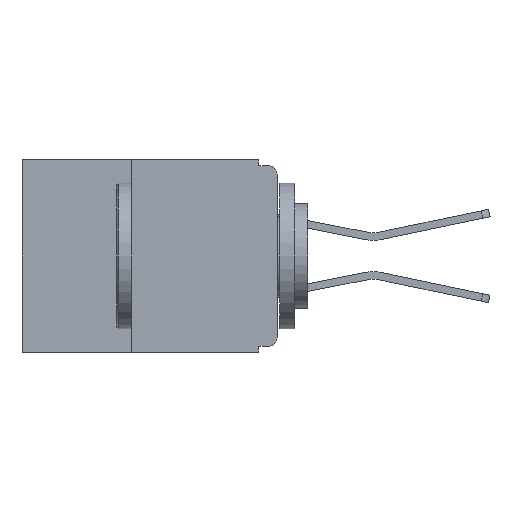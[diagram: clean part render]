
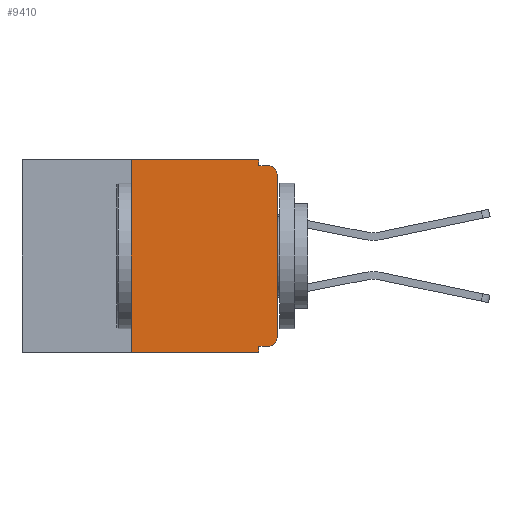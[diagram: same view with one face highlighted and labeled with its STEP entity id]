
A CAD part, left-side view. The second image highlights one B-rep face of the part: STEP entity #9410.
In plain terms, the highlighted planar face has unit normal (-1, 0, 0).
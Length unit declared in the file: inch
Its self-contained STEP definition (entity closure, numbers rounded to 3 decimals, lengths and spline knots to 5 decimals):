
#22 = VECTOR ( 'NONE', #3259, 39.37008 ) ;
#170 = VERTEX_POINT ( 'NONE', #4362 ) ;
#253 = DIRECTION ( 'NONE',  ( 0., 0., -1. ) ) ;
#289 = DIRECTION ( 'NONE',  ( 0., 1., 0. ) ) ;
#506 = VERTEX_POINT ( 'NONE', #2105 ) ;
#507 = EDGE_CURVE ( 'NONE', #8969, #3438, #7579, .T. ) ;
#522 = DIRECTION ( 'NONE',  ( 1., 0., 0. ) ) ;
#640 = EDGE_CURVE ( 'NONE', #170, #8969, #14253, .T. ) ;
#646 = ORIENTED_EDGE ( 'NONE', *, *, #10496, .F. ) ;
#837 = ORIENTED_EDGE ( 'NONE', *, *, #13535, .T. ) ;
#1074 = CARTESIAN_POINT ( 'NONE',  ( 0., 0.031, 0. ) ) ;
#1313 = VERTEX_POINT ( 'NONE', #2822 ) ;
#1616 = ORIENTED_EDGE ( 'NONE', *, *, #4049, .T. ) ;
#1804 = CARTESIAN_POINT ( 'NONE',  ( 0., 0.25, 0. ) ) ;
#1896 = DIRECTION ( 'NONE',  ( 0., 0., 1. ) ) ;
#2105 = CARTESIAN_POINT ( 'NONE',  ( 0., 0.031, -0.32 ) ) ;
#2135 = EDGE_CURVE ( 'NONE', #5074, #9166, #2692, .T. ) ;
#2250 = ORIENTED_EDGE ( 'NONE', *, *, #2135, .T. ) ;
#2692 = CIRCLE ( 'NONE', #13013, 0.015 ) ;
#2728 = PLANE ( 'NONE',  #12878 ) ;
#2822 = CARTESIAN_POINT ( 'NONE',  ( 0., 0.015, -0.01 ) ) ;
#2914 = LINE ( 'NONE', #4872, #8069 ) ;
#2948 = ORIENTED_EDGE ( 'NONE', *, *, #507, .F. ) ;
#3066 = LINE ( 'NONE', #5465, #22 ) ;
#3076 = CARTESIAN_POINT ( 'NONE',  ( 0., 0.031, -0.01 ) ) ;
#3259 = DIRECTION ( 'NONE',  ( 0., 0., -1. ) ) ;
#3438 = VERTEX_POINT ( 'NONE', #1074 ) ;
#3751 = DIRECTION ( 'NONE',  ( 0., -1., 0. ) ) ;
#3814 = CARTESIAN_POINT ( 'NONE',  ( 0., 0.015, -0.305 ) ) ;
#4049 = EDGE_CURVE ( 'NONE', #9166, #13528, #13084, .T. ) ;
#4107 = LINE ( 'NONE', #7011, #6673 ) ;
#4362 = CARTESIAN_POINT ( 'NONE',  ( 0., 0.25, -0.33 ) ) ;
#4366 = ORIENTED_EDGE ( 'NONE', *, *, #640, .F. ) ;
#4523 = ORIENTED_EDGE ( 'NONE', *, *, #6803, .F. ) ;
#4835 = VERTEX_POINT ( 'NONE', #3076 ) ;
#4872 = CARTESIAN_POINT ( 'NONE',  ( 0., 0.437, -0.33 ) ) ;
#5035 = CARTESIAN_POINT ( 'NONE',  ( 0., 0.437, 0. ) ) ;
#5074 = VERTEX_POINT ( 'NONE', #5640 ) ;
#5465 = CARTESIAN_POINT ( 'NONE',  ( 0., 0.031, 0. ) ) ;
#5545 = VECTOR ( 'NONE', #1896, 39.37008 ) ;
#5640 = CARTESIAN_POINT ( 'NONE',  ( 0., 0.015, -0.32 ) ) ;
#5930 = EDGE_CURVE ( 'NONE', #3438, #4835, #3066, .T. ) ;
#6469 = VECTOR ( 'NONE', #9945, 39.37008 ) ;
#6673 = VECTOR ( 'NONE', #289, 39.37008 ) ;
#6803 = EDGE_CURVE ( 'NONE', #5074, #506, #4107, .T. ) ;
#6806 = LINE ( 'NONE', #9896, #6469 ) ;
#6982 = DIRECTION ( 'NONE',  ( -1., 0., 0. ) ) ;
#7011 = CARTESIAN_POINT ( 'NONE',  ( 0., 0., -0.32 ) ) ;
#7251 = VECTOR ( 'NONE', #8173, 39.37008 ) ;
#7579 = LINE ( 'NONE', #10080, #13081 ) ;
#7591 = ORIENTED_EDGE ( 'NONE', *, *, #5930, .F. ) ;
#7895 = CARTESIAN_POINT ( 'NONE',  ( 0., 0., -0.01 ) ) ;
#8069 = VECTOR ( 'NONE', #3751, 39.37008 ) ;
#8170 = VECTOR ( 'NONE', #9019, 39.37008 ) ;
#8173 = DIRECTION ( 'NONE',  ( 0., 0., 1. ) ) ;
#8320 = DIRECTION ( 'NONE',  ( 0., 0., -1. ) ) ;
#8385 = EDGE_CURVE ( 'NONE', #506, #12043, #6806, .T. ) ;
#8523 = LINE ( 'NONE', #7895, #8170 ) ;
#8678 = EDGE_LOOP ( 'NONE', ( #1616, #11404, #646, #7591, #2948, #4366, #837, #13991, #4523, #2250 ) ) ;
#8726 = CARTESIAN_POINT ( 'NONE',  ( 0., 0.031, -0.33 ) ) ;
#8924 = DIRECTION ( 'NONE',  ( 0., -1., 0. ) ) ;
#8969 = VERTEX_POINT ( 'NONE', #1804 ) ;
#9019 = DIRECTION ( 'NONE',  ( 0., -1., 0. ) ) ;
#9166 = VERTEX_POINT ( 'NONE', #13366 ) ;
#9326 = DIRECTION ( 'NONE',  ( -1., 0., 0. ) ) ;
#9410 = ADVANCED_FACE ( 'NONE', ( #10919 ), #2728, .F. ) ;
#9510 = CARTESIAN_POINT ( 'NONE',  ( 0., 0.25, -0.33 ) ) ;
#9665 = DIRECTION ( 'NONE',  ( 0., 0., -1. ) ) ;
#9896 = CARTESIAN_POINT ( 'NONE',  ( 0., 0.031, -0.33 ) ) ;
#9945 = DIRECTION ( 'NONE',  ( 0., 0., -1. ) ) ;
#10080 = CARTESIAN_POINT ( 'NONE',  ( 0., 0.437, 0. ) ) ;
#10496 = EDGE_CURVE ( 'NONE', #4835, #1313, #8523, .T. ) ;
#10919 = FACE_OUTER_BOUND ( 'NONE', #8678, .T. ) ;
#11404 = ORIENTED_EDGE ( 'NONE', *, *, #11756, .T. ) ;
#11434 = CARTESIAN_POINT ( 'NONE',  ( 0., 0., -0.025 ) ) ;
#11756 = EDGE_CURVE ( 'NONE', #13528, #1313, #14302, .T. ) ;
#12043 = VERTEX_POINT ( 'NONE', #8726 ) ;
#12878 = AXIS2_PLACEMENT_3D ( 'NONE', #5035, #522, #8320 ) ;
#13013 = AXIS2_PLACEMENT_3D ( 'NONE', #3814, #9326, #9665 ) ;
#13081 = VECTOR ( 'NONE', #8924, 39.37008 ) ;
#13084 = LINE ( 'NONE', #13844, #7251 ) ;
#13297 = AXIS2_PLACEMENT_3D ( 'NONE', #13536, #6982, #253 ) ;
#13366 = CARTESIAN_POINT ( 'NONE',  ( 0., 0., -0.305 ) ) ;
#13528 = VERTEX_POINT ( 'NONE', #11434 ) ;
#13535 = EDGE_CURVE ( 'NONE', #170, #12043, #2914, .T. ) ;
#13536 = CARTESIAN_POINT ( 'NONE',  ( 0., 0.015, -0.025 ) ) ;
#13844 = CARTESIAN_POINT ( 'NONE',  ( 0., 0., 0. ) ) ;
#13991 = ORIENTED_EDGE ( 'NONE', *, *, #8385, .F. ) ;
#14253 = LINE ( 'NONE', #9510, #5545 ) ;
#14302 = CIRCLE ( 'NONE', #13297, 0.015 ) ;
